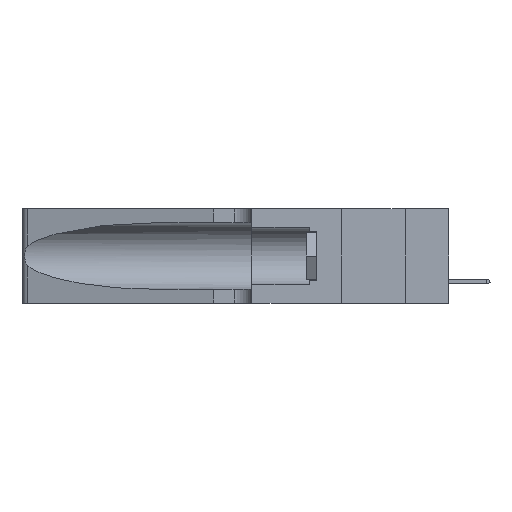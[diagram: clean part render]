
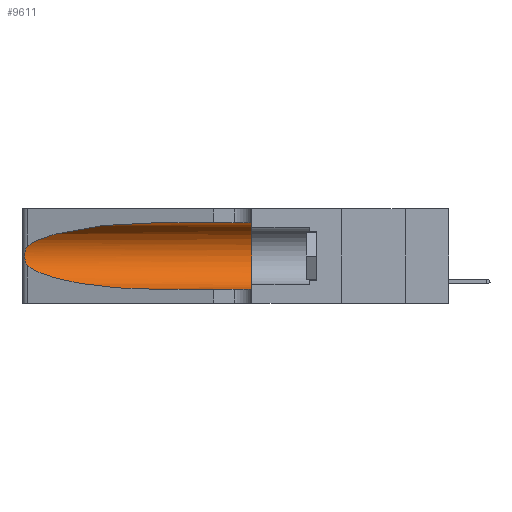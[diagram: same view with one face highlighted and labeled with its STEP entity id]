
A CAD part, left-side view. The second image highlights one B-rep face of the part: STEP entity #9611.
In plain terms, the highlighted cylindrical face has radius 3.308 mm (diameter 6.617 mm), a partial arc.
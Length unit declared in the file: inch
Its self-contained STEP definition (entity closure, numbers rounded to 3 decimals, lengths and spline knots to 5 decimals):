
#441 = CARTESIAN_POINT ( 'NONE',  ( 0.1305, 0.35, 0.31525 ) ) ;
#2312 = CARTESIAN_POINT ( 'NONE',  ( 0.1305, 0.72297, 0.31525 ) ) ;
#3982 = LINE ( 'NONE', #15240, #18109 ) ;
#4124 = CARTESIAN_POINT ( 'NONE',  ( 0.26018, 1.23835, 0.19895 ) ) ;
#4259 = CARTESIAN_POINT ( 'NONE',  ( 0.1305, 0.35, 0.05475 ) ) ;
#4369 = EDGE_CURVE ( 'NONE', #8366, #17185, #14851, .T. ) ;
#4509 = ORIENTED_EDGE ( 'NONE', *, *, #21606, .T. ) ;
#4891 = EDGE_CURVE ( 'NONE', #15091, #8366, #3982, .T. ) ;
#5165 = CYLINDRICAL_SURFACE ( 'NONE', #12398, 0.13025 ) ;
#5579 = CARTESIAN_POINT ( 'NONE',  ( 0.1305, 0.72297, 0.05475 ) ) ;
#6878 = CARTESIAN_POINT ( 'NONE',  ( 0.1305, 1.61858, 0.185 ) ) ;
#6952 = DIRECTION ( 'NONE',  ( 0., -1., 0. ) ) ;
#7395 = CARTESIAN_POINT ( 'NONE',  ( 0.18966, 0.96281, 0.31525 ) ) ;
#7683 = CARTESIAN_POINT ( 'NONE',  ( 0.25639, 1.23186, 0.15144 ) ) ;
#7860 =( BOUNDED_CURVE ( )  B_SPLINE_CURVE ( 3, ( #2312, #7395, #12994, #12830 ),
 .UNSPECIFIED., .F., .F. ) 
 B_SPLINE_CURVE_WITH_KNOTS ( ( 4, 4 ),
 ( 1.5708, 2.84003 ),
 .UNSPECIFIED. ) 
 CURVE ( )  GEOMETRIC_REPRESENTATION_ITEM ( )  RATIONAL_B_SPLINE_CURVE ( ( 1., 0.87, 0.87, 1. ) ) 
 REPRESENTATION_ITEM ( '' )  );
#7882 = EDGE_CURVE ( 'NONE', #14090, #18545, #15953, .T. ) ;
#8204 = FACE_OUTER_BOUND ( 'NONE', #20461, .T. ) ;
#8366 = VERTEX_POINT ( 'NONE', #441 ) ;
#8488 = LINE ( 'NONE', #12708, #10167 ) ;
#9083 = CARTESIAN_POINT ( 'NONE',  ( 0.25555, 1.22993, 0.14849 ) ) ;
#9089 = CARTESIAN_POINT ( 'NONE',  ( 0.25487, 1.22718, 0.14631 ) ) ;
#9395 = CARTESIAN_POINT ( 'NONE',  ( 0.25854, 1.2359, 0.20912 ) ) ;
#9599 = CARTESIAN_POINT ( 'NONE',  ( 0.1305, 0.35, 0.185 ) ) ;
#9611 = ADVANCED_FACE ( 'NONE', ( #8204 ), #5165, .F. ) ;
#9802 = EDGE_CURVE ( 'NONE', #20307, #17185, #8488, .T. ) ;
#10167 = VECTOR ( 'NONE', #21548, 39.37008 ) ;
#10556 =( BOUNDED_CURVE ( )  B_SPLINE_CURVE ( 3, ( #9089, #19490, #17907, #21568 ),
 .UNSPECIFIED., .F., .F. ) 
 B_SPLINE_CURVE_WITH_KNOTS ( ( 4, 4 ),
 ( 3.44316, 4.71239 ),
 .UNSPECIFIED. ) 
 CURVE ( )  GEOMETRIC_REPRESENTATION_ITEM ( )  RATIONAL_B_SPLINE_CURVE ( ( 1., 0.87, 0.87, 1. ) ) 
 REPRESENTATION_ITEM ( '' )  );
#10968 = ORIENTED_EDGE ( 'NONE', *, *, #9802, .T. ) ;
#11163 = ORIENTED_EDGE ( 'NONE', *, *, #18925, .T. ) ;
#11184 = CARTESIAN_POINT ( 'NONE',  ( 0.25487, 1.22718, 0.22369 ) ) ;
#11530 = AXIS2_PLACEMENT_3D ( 'NONE', #9599, #16483, #12919 ) ;
#12015 = CARTESIAN_POINT ( 'NONE',  ( 0.25487, 1.22718, 0.14631 ) ) ;
#12398 = AXIS2_PLACEMENT_3D ( 'NONE', #6878, #6952, #22684 ) ;
#12708 = CARTESIAN_POINT ( 'NONE',  ( 0.1305, 1.61858, 0.05475 ) ) ;
#12830 = CARTESIAN_POINT ( 'NONE',  ( 0.25487, 1.22718, 0.22369 ) ) ;
#12872 = CARTESIAN_POINT ( 'NONE',  ( 0.26075, 1.23896, 0.19203 ) ) ;
#12919 = DIRECTION ( 'NONE',  ( 0., 0., 1. ) ) ;
#12960 = CARTESIAN_POINT ( 'NONE',  ( 0.25639, 1.23184, 0.21858 ) ) ;
#12994 = CARTESIAN_POINT ( 'NONE',  ( 0.2373, 1.15595, 0.28018 ) ) ;
#13493 = ORIENTED_EDGE ( 'NONE', *, *, #7882, .T. ) ;
#13537 = DIRECTION ( 'NONE',  ( 0., -1., 0. ) ) ;
#14090 = VERTEX_POINT ( 'NONE', #14685 ) ;
#14593 = CARTESIAN_POINT ( 'NONE',  ( 0.25555, 1.22994, 0.2215 ) ) ;
#14623 = ORIENTED_EDGE ( 'NONE', *, *, #4369, .F. ) ;
#14685 = CARTESIAN_POINT ( 'NONE',  ( 0.25487, 1.22718, 0.22369 ) ) ;
#14851 = CIRCLE ( 'NONE', #11530, 0.13025 ) ;
#15091 = VERTEX_POINT ( 'NONE', #18092 ) ;
#15240 = CARTESIAN_POINT ( 'NONE',  ( 0.1305, 1.61858, 0.31525 ) ) ;
#15953 = B_SPLINE_CURVE_WITH_KNOTS ( 'NONE', 3,
 ( #11184, #14593, #12960, #19947, #9395, #4124, #12872, #17981, #16364, #18295, #19716, #7683, #9083, #18133 ),
 .UNSPECIFIED., .F., .F.,
 ( 4, 2, 2, 2, 2, 2, 4 ),
 ( 0., 0.00027, 0.00053, 0.00107, 0.0016, 0.00187, 0.00214 ),
 .UNSPECIFIED. ) ;
#16115 = ORIENTED_EDGE ( 'NONE', *, *, #4891, .F. ) ;
#16364 = CARTESIAN_POINT ( 'NONE',  ( 0.26017, 1.23833, 0.17102 ) ) ;
#16483 = DIRECTION ( 'NONE',  ( 0., 1., 0. ) ) ;
#17185 = VERTEX_POINT ( 'NONE', #4259 ) ;
#17907 = CARTESIAN_POINT ( 'NONE',  ( 0.18966, 0.96281, 0.05475 ) ) ;
#17981 = CARTESIAN_POINT ( 'NONE',  ( 0.26075, 1.23896, 0.178 ) ) ;
#18092 = CARTESIAN_POINT ( 'NONE',  ( 0.1305, 0.72297, 0.31525 ) ) ;
#18109 = VECTOR ( 'NONE', #13537, 39.37008 ) ;
#18133 = CARTESIAN_POINT ( 'NONE',  ( 0.25487, 1.22718, 0.14631 ) ) ;
#18295 = CARTESIAN_POINT ( 'NONE',  ( 0.25856, 1.23593, 0.16098 ) ) ;
#18545 = VERTEX_POINT ( 'NONE', #12015 ) ;
#18925 = EDGE_CURVE ( 'NONE', #18545, #20307, #10556, .T. ) ;
#19490 = CARTESIAN_POINT ( 'NONE',  ( 0.2373, 1.15595, 0.08982 ) ) ;
#19716 = CARTESIAN_POINT ( 'NONE',  ( 0.25789, 1.23486, 0.15765 ) ) ;
#19947 = CARTESIAN_POINT ( 'NONE',  ( 0.25787, 1.23484, 0.2124 ) ) ;
#20307 = VERTEX_POINT ( 'NONE', #5579 ) ;
#20461 = EDGE_LOOP ( 'NONE', ( #4509, #13493, #11163, #10968, #14623, #16115 ) ) ;
#21548 = DIRECTION ( 'NONE',  ( 0., -1., 0. ) ) ;
#21568 = CARTESIAN_POINT ( 'NONE',  ( 0.1305, 0.72297, 0.05475 ) ) ;
#21606 = EDGE_CURVE ( 'NONE', #15091, #14090, #7860, .T. ) ;
#22684 = DIRECTION ( 'NONE',  ( 0., 0., -1. ) ) ;
